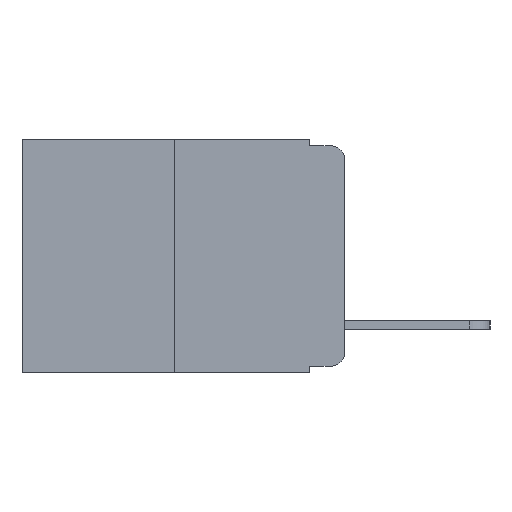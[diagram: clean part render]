
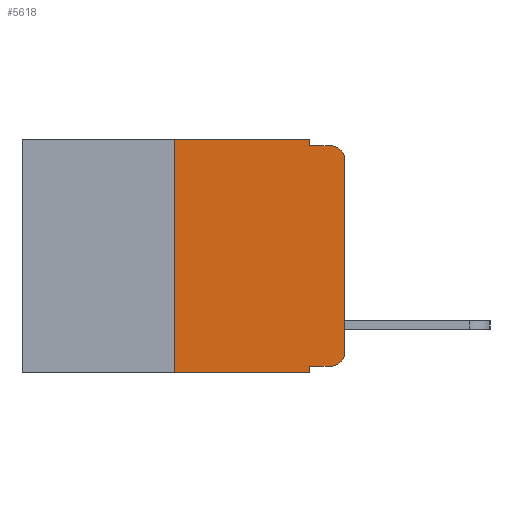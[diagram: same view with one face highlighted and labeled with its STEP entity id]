
A CAD part, left-side view. The second image highlights one B-rep face of the part: STEP entity #5618.
In plain terms, the highlighted planar face has unit normal (-1, 0, 0).
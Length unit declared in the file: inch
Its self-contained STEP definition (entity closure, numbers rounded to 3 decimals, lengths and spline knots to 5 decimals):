
#106 = ORIENTED_EDGE ( 'NONE', *, *, #11210, .F. ) ;
#173 = CARTESIAN_POINT ( 'NONE',  ( 0., 0.051, 0. ) ) ;
#214 = VERTEX_POINT ( 'NONE', #6537 ) ;
#389 = EDGE_CURVE ( 'NONE', #10890, #2795, #815, .T. ) ;
#473 = ORIENTED_EDGE ( 'NONE', *, *, #11025, .F. ) ;
#584 = ORIENTED_EDGE ( 'NONE', *, *, #10830, .T. ) ;
#815 = LINE ( 'NONE', #1791, #11005 ) ;
#852 = ORIENTED_EDGE ( 'NONE', *, *, #10612, .T. ) ;
#870 = VERTEX_POINT ( 'NONE', #6577 ) ;
#1267 = AXIS2_PLACEMENT_3D ( 'NONE', #12218, #12052, #11832 ) ;
#1330 = VERTEX_POINT ( 'NONE', #4305 ) ;
#1337 = CARTESIAN_POINT ( 'NONE',  ( 0., 0.25, 0. ) ) ;
#1457 = VERTEX_POINT ( 'NONE', #8250 ) ;
#1735 = CIRCLE ( 'NONE', #1267, 0.02 ) ;
#1791 = CARTESIAN_POINT ( 'NONE',  ( 0., 0.473, 0. ) ) ;
#2167 = VECTOR ( 'NONE', #7417, 39.37008 ) ;
#2324 = DIRECTION ( 'NONE',  ( -1., 0., 0. ) ) ;
#2343 = DIRECTION ( 'NONE',  ( 0., 0., -1. ) ) ;
#2346 = CARTESIAN_POINT ( 'NONE',  ( 0., 0.02, -0.03 ) ) ;
#2686 = VECTOR ( 'NONE', #6447, 39.37008 ) ;
#2795 = VERTEX_POINT ( 'NONE', #14004 ) ;
#3163 = LINE ( 'NONE', #6279, #2686 ) ;
#3457 = CARTESIAN_POINT ( 'NONE',  ( 0., 0.02, -0.01 ) ) ;
#3688 = VECTOR ( 'NONE', #5824, 39.37008 ) ;
#4305 = CARTESIAN_POINT ( 'NONE',  ( 0., 0.25, -0.343 ) ) ;
#5113 = DIRECTION ( 'NONE',  ( 0., -1., 0. ) ) ;
#5312 = VERTEX_POINT ( 'NONE', #6240 ) ;
#5618 = ADVANCED_FACE ( 'NONE', ( #11949 ), #12339, .F. ) ;
#5800 = CARTESIAN_POINT ( 'NONE',  ( 0., 0., 0. ) ) ;
#5824 = DIRECTION ( 'NONE',  ( 0., 0., 1. ) ) ;
#6240 = CARTESIAN_POINT ( 'NONE',  ( 0., 0.051, -0.333 ) ) ;
#6279 = CARTESIAN_POINT ( 'NONE',  ( 0., 0.25, 0. ) ) ;
#6432 = LINE ( 'NONE', #6581, #2167 ) ;
#6447 = DIRECTION ( 'NONE',  ( 0., 0., 1. ) ) ;
#6514 = VECTOR ( 'NONE', #15706, 39.37008 ) ;
#6537 = CARTESIAN_POINT ( 'NONE',  ( 0., 0.02, -0.333 ) ) ;
#6577 = CARTESIAN_POINT ( 'NONE',  ( 0., 0.051, -0.01 ) ) ;
#6581 = CARTESIAN_POINT ( 'NONE',  ( 0., 0.473, -0.343 ) ) ;
#6625 = VERTEX_POINT ( 'NONE', #15362 ) ;
#7417 = DIRECTION ( 'NONE',  ( 0., -1., 0. ) ) ;
#8239 = LINE ( 'NONE', #5800, #3688 ) ;
#8250 = CARTESIAN_POINT ( 'NONE',  ( 0., 0., -0.03 ) ) ;
#9059 = VECTOR ( 'NONE', #14599, 39.37008 ) ;
#10419 = VECTOR ( 'NONE', #14280, 39.37008 ) ;
#10612 = EDGE_CURVE ( 'NONE', #13304, #1457, #8239, .T. ) ;
#10830 = EDGE_CURVE ( 'NONE', #1457, #15271, #15976, .T. ) ;
#10890 = VERTEX_POINT ( 'NONE', #1337 ) ;
#11005 = VECTOR ( 'NONE', #5113, 39.37008 ) ;
#11025 = EDGE_CURVE ( 'NONE', #870, #15271, #16129, .T. ) ;
#11198 = AXIS2_PLACEMENT_3D ( 'NONE', #14305, #13005, #12956 ) ;
#11210 = EDGE_CURVE ( 'NONE', #2795, #870, #12302, .T. ) ;
#11746 = AXIS2_PLACEMENT_3D ( 'NONE', #2346, #2324, #2343 ) ;
#11832 = DIRECTION ( 'NONE',  ( 0., 0., -1. ) ) ;
#11949 = FACE_OUTER_BOUND ( 'NONE', #16461, .T. ) ;
#12052 = DIRECTION ( 'NONE',  ( -1., 0., 0. ) ) ;
#12218 = CARTESIAN_POINT ( 'NONE',  ( 0., 0.02, -0.313 ) ) ;
#12302 = LINE ( 'NONE', #14501, #9059 ) ;
#12339 = PLANE ( 'NONE',  #11198 ) ;
#12393 = ORIENTED_EDGE ( 'NONE', *, *, #13319, .T. ) ;
#12501 = ORIENTED_EDGE ( 'NONE', *, *, #13266, .T. ) ;
#12621 = ORIENTED_EDGE ( 'NONE', *, *, #13247, .F. ) ;
#12754 = EDGE_CURVE ( 'NONE', #1330, #10890, #3163, .T. ) ;
#12956 = DIRECTION ( 'NONE',  ( 0., 0., -1. ) ) ;
#12992 = ORIENTED_EDGE ( 'NONE', *, *, #15793, .T. ) ;
#13005 = DIRECTION ( 'NONE',  ( 1., 0., 0. ) ) ;
#13089 = ORIENTED_EDGE ( 'NONE', *, *, #12754, .F. ) ;
#13182 = VECTOR ( 'NONE', #15274, 39.37008 ) ;
#13247 = EDGE_CURVE ( 'NONE', #5312, #6625, #16416, .T. ) ;
#13266 = EDGE_CURVE ( 'NONE', #5312, #214, #16087, .T. ) ;
#13285 = ORIENTED_EDGE ( 'NONE', *, *, #389, .F. ) ;
#13304 = VERTEX_POINT ( 'NONE', #13873 ) ;
#13319 = EDGE_CURVE ( 'NONE', #214, #13304, #1735, .T. ) ;
#13873 = CARTESIAN_POINT ( 'NONE',  ( 0., 0., -0.313 ) ) ;
#14004 = CARTESIAN_POINT ( 'NONE',  ( 0., 0.051, 0. ) ) ;
#14280 = DIRECTION ( 'NONE',  ( 0., -1., 0. ) ) ;
#14305 = CARTESIAN_POINT ( 'NONE',  ( 0., 0.473, 0. ) ) ;
#14501 = CARTESIAN_POINT ( 'NONE',  ( 0., 0.051, 0. ) ) ;
#14599 = DIRECTION ( 'NONE',  ( 0., 0., -1. ) ) ;
#15271 = VERTEX_POINT ( 'NONE', #3457 ) ;
#15274 = DIRECTION ( 'NONE',  ( 0., 0., -1. ) ) ;
#15362 = CARTESIAN_POINT ( 'NONE',  ( 0., 0.051, -0.343 ) ) ;
#15706 = DIRECTION ( 'NONE',  ( 0., -1., 0. ) ) ;
#15748 = CARTESIAN_POINT ( 'NONE',  ( 0., 0.051, -0.01 ) ) ;
#15793 = EDGE_CURVE ( 'NONE', #1330, #6625, #6432, .T. ) ;
#15976 = CIRCLE ( 'NONE', #11746, 0.02 ) ;
#16087 = LINE ( 'NONE', #16211, #10419 ) ;
#16129 = LINE ( 'NONE', #15748, #6514 ) ;
#16211 = CARTESIAN_POINT ( 'NONE',  ( 0., 0.051, -0.333 ) ) ;
#16416 = LINE ( 'NONE', #173, #13182 ) ;
#16461 = EDGE_LOOP ( 'NONE', ( #852, #584, #473, #106, #13285, #13089, #12992, #12621, #12501, #12393 ) ) ;
